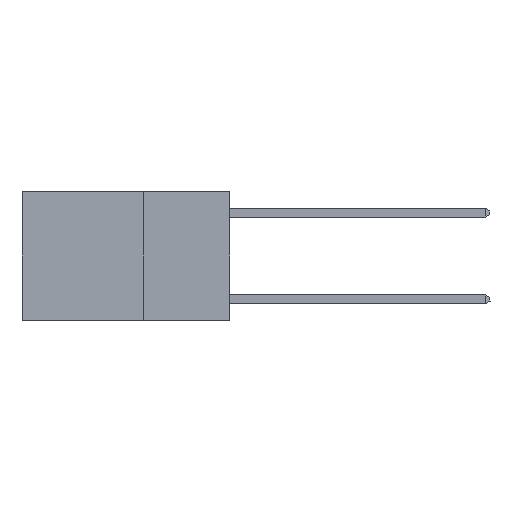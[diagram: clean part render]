
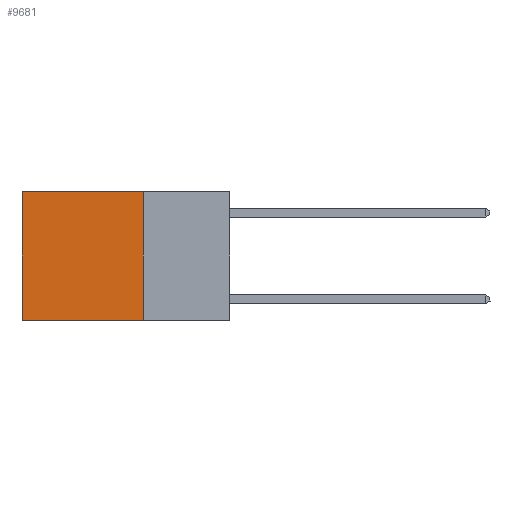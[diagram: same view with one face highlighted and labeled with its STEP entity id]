
A CAD part, left-side view. The second image highlights one B-rep face of the part: STEP entity #9681.
In plain terms, the highlighted planar face has unit normal (-1, 0, 0).
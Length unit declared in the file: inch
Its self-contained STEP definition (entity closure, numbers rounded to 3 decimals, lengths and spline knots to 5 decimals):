
#46 = CARTESIAN_POINT ( 'NONE',  ( 0.2625, 0.6, 0. ) ) ;
#591 = VECTOR ( 'NONE', #12803, 39.37008 ) ;
#646 = CARTESIAN_POINT ( 'NONE',  ( 0.2625, 0.25, 0. ) ) ;
#987 = LINE ( 'NONE', #13163, #13899 ) ;
#1153 = DIRECTION ( 'NONE',  ( 0., 1., 0. ) ) ;
#1982 = DIRECTION ( 'NONE',  ( 0., 0., -1. ) ) ;
#3435 = DIRECTION ( 'NONE',  ( 0., 1., 0. ) ) ;
#4073 = CARTESIAN_POINT ( 'NONE',  ( 0.2625, 0.25, -0.37 ) ) ;
#4276 = ORIENTED_EDGE ( 'NONE', *, *, #7694, .T. ) ;
#5223 = CARTESIAN_POINT ( 'NONE',  ( 0.2625, 0.25, 0. ) ) ;
#6661 = AXIS2_PLACEMENT_3D ( 'NONE', #9385, #26405, #23498 ) ;
#7486 = VERTEX_POINT ( 'NONE', #20132 ) ;
#7535 = VERTEX_POINT ( 'NONE', #5223 ) ;
#7688 = EDGE_CURVE ( 'NONE', #7729, #7486, #7979, .T. ) ;
#7694 = EDGE_CURVE ( 'NONE', #7535, #31972, #987, .T. ) ;
#7729 = VERTEX_POINT ( 'NONE', #4073 ) ;
#7849 = ORIENTED_EDGE ( 'NONE', *, *, #7688, .F. ) ;
#7979 = LINE ( 'NONE', #12831, #27873 ) ;
#9385 = CARTESIAN_POINT ( 'NONE',  ( 0.2625, 0.25, 0. ) ) ;
#9681 = ADVANCED_FACE ( 'NONE', ( #31427 ), #14092, .F. ) ;
#12803 = DIRECTION ( 'NONE',  ( 0., 0., -1. ) ) ;
#12831 = CARTESIAN_POINT ( 'NONE',  ( 0.2625, 0.25, -0.37 ) ) ;
#13163 = CARTESIAN_POINT ( 'NONE',  ( 0.2625, 0.25, 0. ) ) ;
#13899 = VECTOR ( 'NONE', #1153, 39.37008 ) ;
#14092 = PLANE ( 'NONE',  #6661 ) ;
#15253 = LINE ( 'NONE', #646, #591 ) ;
#15295 = VECTOR ( 'NONE', #1982, 39.37008 ) ;
#15923 = ORIENTED_EDGE ( 'NONE', *, *, #30104, .T. ) ;
#16752 = LINE ( 'NONE', #26634, #15295 ) ;
#20132 = CARTESIAN_POINT ( 'NONE',  ( 0.2625, 0.6, -0.37 ) ) ;
#21678 = ORIENTED_EDGE ( 'NONE', *, *, #23670, .F. ) ;
#23498 = DIRECTION ( 'NONE',  ( 0., 0., -1. ) ) ;
#23609 = EDGE_LOOP ( 'NONE', ( #15923, #7849, #21678, #4276 ) ) ;
#23670 = EDGE_CURVE ( 'NONE', #7535, #7729, #15253, .T. ) ;
#26405 = DIRECTION ( 'NONE',  ( 1., 0., 0. ) ) ;
#26634 = CARTESIAN_POINT ( 'NONE',  ( 0.2625, 0.6, 0. ) ) ;
#27873 = VECTOR ( 'NONE', #3435, 39.37008 ) ;
#30104 = EDGE_CURVE ( 'NONE', #31972, #7486, #16752, .T. ) ;
#31427 = FACE_OUTER_BOUND ( 'NONE', #23609, .T. ) ;
#31972 = VERTEX_POINT ( 'NONE', #46 ) ;
